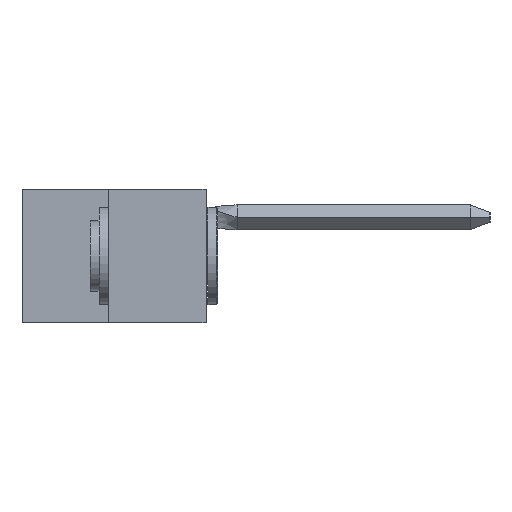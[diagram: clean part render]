
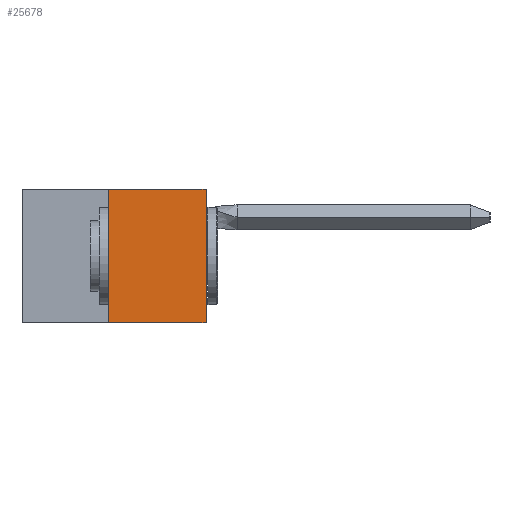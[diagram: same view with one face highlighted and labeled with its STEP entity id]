
A CAD part, left-side view. The second image highlights one B-rep face of the part: STEP entity #25678.
In plain terms, the highlighted planar face has unit normal (-1, 0, 0).
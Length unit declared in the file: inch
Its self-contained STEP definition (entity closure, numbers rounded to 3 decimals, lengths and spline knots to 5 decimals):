
#905 = VERTEX_POINT ( 'NONE', #14863 ) ;
#1005 = DIRECTION ( 'NONE',  ( 0., 0., 1. ) ) ;
#1181 = ORIENTED_EDGE ( 'NONE', *, *, #1419, .T. ) ;
#1419 = EDGE_CURVE ( 'NONE', #22536, #18480, #13305, .T. ) ;
#2205 = DIRECTION ( 'NONE',  ( 1., 0., 0. ) ) ;
#2984 = EDGE_CURVE ( 'NONE', #26904, #905, #28601, .T. ) ;
#4299 = FACE_OUTER_BOUND ( 'NONE', #6345, .T. ) ;
#4611 = PLANE ( 'NONE',  #26066 ) ;
#6345 = EDGE_LOOP ( 'NONE', ( #26524, #29572, #8215, #1181 ) ) ;
#6959 = CARTESIAN_POINT ( 'NONE',  ( 0., 0.473, 0. ) ) ;
#7288 = VECTOR ( 'NONE', #9085, 39.37008 ) ;
#7397 = CARTESIAN_POINT ( 'NONE',  ( 0., 0.25, -0.343 ) ) ;
#8215 = ORIENTED_EDGE ( 'NONE', *, *, #24152, .T. ) ;
#9085 = DIRECTION ( 'NONE',  ( 0., 0., 1. ) ) ;
#10111 = VECTOR ( 'NONE', #1005, 39.37008 ) ;
#10230 = CARTESIAN_POINT ( 'NONE',  ( 0., 0., 0. ) ) ;
#12565 = EDGE_CURVE ( 'NONE', #905, #18480, #13649, .T. ) ;
#13305 = LINE ( 'NONE', #19277, #10111 ) ;
#13649 = LINE ( 'NONE', #6959, #14438 ) ;
#14438 = VECTOR ( 'NONE', #21902, 39.37008 ) ;
#14863 = CARTESIAN_POINT ( 'NONE',  ( 0., 0.25, 0. ) ) ;
#17409 = CARTESIAN_POINT ( 'NONE',  ( 0., 0., -0.343 ) ) ;
#18480 = VERTEX_POINT ( 'NONE', #10230 ) ;
#19277 = CARTESIAN_POINT ( 'NONE',  ( 0., 0., 0. ) ) ;
#19382 = CARTESIAN_POINT ( 'NONE',  ( 0., 0.25, 0. ) ) ;
#21902 = DIRECTION ( 'NONE',  ( 0., -1., 0. ) ) ;
#22242 = DIRECTION ( 'NONE',  ( 0., -1., 0. ) ) ;
#22536 = VERTEX_POINT ( 'NONE', #17409 ) ;
#24152 = EDGE_CURVE ( 'NONE', #26904, #22536, #32424, .T. ) ;
#24204 = VECTOR ( 'NONE', #22242, 39.37008 ) ;
#24573 = CARTESIAN_POINT ( 'NONE',  ( 0., 0.473, 0. ) ) ;
#24796 = CARTESIAN_POINT ( 'NONE',  ( 0., 0.473, -0.343 ) ) ;
#24995 = DIRECTION ( 'NONE',  ( 0., 0., -1. ) ) ;
#25678 = ADVANCED_FACE ( 'NONE', ( #4299 ), #4611, .F. ) ;
#26066 = AXIS2_PLACEMENT_3D ( 'NONE', #24573, #2205, #24995 ) ;
#26524 = ORIENTED_EDGE ( 'NONE', *, *, #12565, .F. ) ;
#26904 = VERTEX_POINT ( 'NONE', #7397 ) ;
#28601 = LINE ( 'NONE', #19382, #7288 ) ;
#29572 = ORIENTED_EDGE ( 'NONE', *, *, #2984, .F. ) ;
#32424 = LINE ( 'NONE', #24796, #24204 ) ;
